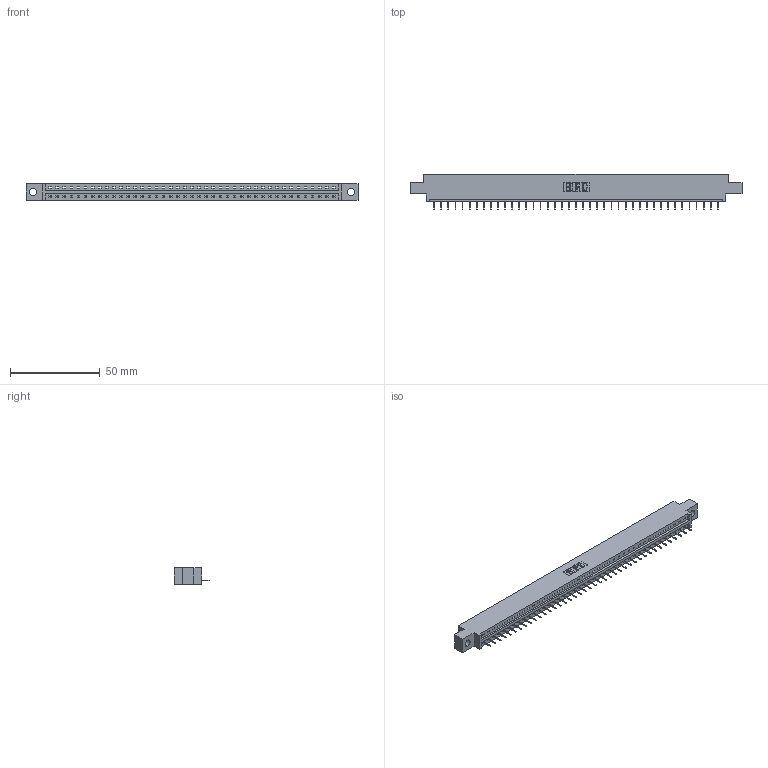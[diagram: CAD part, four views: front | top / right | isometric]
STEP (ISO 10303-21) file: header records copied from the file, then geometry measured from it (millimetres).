
FILE_DESCRIPTION (( 'STEP AP203' ), '1' );
FILE_NAME ('387-041-524-604.STEP', '2018-09-19T18:06:06', ( '' ), ( '' ), 'SwSTEP 2.0', 'SolidWorks 2016', '' );
FILE_SCHEMA (( 'CONFIG_CONTROL_DESIGN' ));
Length unit declared in the file: inch
Products named in the file (3): 337 Part_0.170 Offset - 0.156 Dia-TH; 345-292-001_345-293-124; 387-041-524-604
Assembly tree (42 placements, depth 2):
  387-041-524-604
    337 Part_0.170 Offset - 0.156 Dia-TH
    345-292-001_345-293-124  x41
Bounding box: 185.47 x 19.69 x 9.4 mm (x, y, z)
Volume: 18896.7 mm3; surface area: 18843.6 mm2
Topology: 42 solids, 42 shells, 2824 faces, 8195 edges, 5298 vertices
Faces by surface type: plane 2206, cylinder 618
Entity records: 30815 total; most frequent: CARTESIAN_POINT 5373, ORIENTED_EDGE 5350, DIRECTION 4525, EDGE_CURVE 2675, LINE 2551, VECTOR 2551, VERTEX_POINT 1778, AXIS2_PLACEMENT_3D 987
